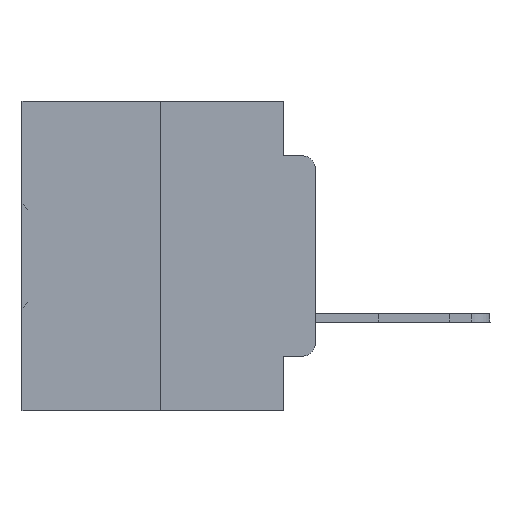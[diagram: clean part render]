
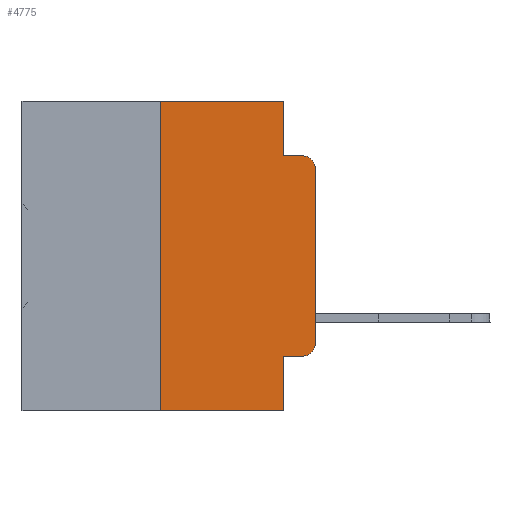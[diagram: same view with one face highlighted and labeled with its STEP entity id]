
A CAD part, left-side view. The second image highlights one B-rep face of the part: STEP entity #4775.
In plain terms, the highlighted planar face has unit normal (-1, 0, 0).
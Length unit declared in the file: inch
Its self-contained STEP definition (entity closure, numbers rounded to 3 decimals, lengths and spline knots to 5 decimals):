
#44 = CARTESIAN_POINT ( 'NONE',  ( 0., 0.25, 0. ) ) ;
#73 = EDGE_CURVE ( 'NONE', #25052, #33834, #27180, .T. ) ;
#574 = VECTOR ( 'NONE', #32646, 39.37008 ) ;
#826 = DIRECTION ( 'NONE',  ( 0., 0., -1. ) ) ;
#978 = ORIENTED_EDGE ( 'NONE', *, *, #10420, .T. ) ;
#1211 = ORIENTED_EDGE ( 'NONE', *, *, #73, .F. ) ;
#1350 = VECTOR ( 'NONE', #23883, 39.37008 ) ;
#1943 = CARTESIAN_POINT ( 'NONE',  ( 0., 0.02, -0.0885 ) ) ;
#2237 = VECTOR ( 'NONE', #25882, 39.37008 ) ;
#2871 = CIRCLE ( 'NONE', #24149, 0.02 ) ;
#3865 = EDGE_CURVE ( 'NONE', #33834, #7707, #8281, .T. ) ;
#3898 = DIRECTION ( 'NONE',  ( 0., 0., -1. ) ) ;
#4092 = PLANE ( 'NONE',  #24202 ) ;
#4153 = CARTESIAN_POINT ( 'NONE',  ( 0., 0.051, 0. ) ) ;
#4378 = VECTOR ( 'NONE', #26690, 39.37008 ) ;
#4775 = ADVANCED_FACE ( 'NONE', ( #29833 ), #4092, .F. ) ;
#5383 = ORIENTED_EDGE ( 'NONE', *, *, #3865, .F. ) ;
#5728 = EDGE_CURVE ( 'NONE', #25775, #24258, #17668, .T. ) ;
#5816 = CARTESIAN_POINT ( 'NONE',  ( 0., 0., -0.1085 ) ) ;
#6337 = CARTESIAN_POINT ( 'NONE',  ( 0., 0.473, 0. ) ) ;
#6495 = ORIENTED_EDGE ( 'NONE', *, *, #21046, .T. ) ;
#6619 = CARTESIAN_POINT ( 'NONE',  ( 0., 0.02, -0.1085 ) ) ;
#7337 = ORIENTED_EDGE ( 'NONE', *, *, #22895, .T. ) ;
#7707 = VERTEX_POINT ( 'NONE', #32157 ) ;
#7719 = VERTEX_POINT ( 'NONE', #21350 ) ;
#7799 = CARTESIAN_POINT ( 'NONE',  ( 0., 0.473, 0. ) ) ;
#8281 = LINE ( 'NONE', #7799, #574 ) ;
#9077 = VERTEX_POINT ( 'NONE', #23490 ) ;
#9442 = VECTOR ( 'NONE', #17511, 39.37008 ) ;
#9446 = LINE ( 'NONE', #31893, #1350 ) ;
#9457 = EDGE_LOOP ( 'NONE', ( #13786, #6495, #19389, #30653, #5383, #1211, #7337, #30926, #978, #21775 ) ) ;
#10019 = CIRCLE ( 'NONE', #19661, 0.02 ) ;
#10065 = VECTOR ( 'NONE', #32995, 39.37008 ) ;
#10070 = CARTESIAN_POINT ( 'NONE',  ( 0., 0., -0.3915 ) ) ;
#10420 = EDGE_CURVE ( 'NONE', #19494, #7719, #27631, .T. ) ;
#12389 = EDGE_CURVE ( 'NONE', #7707, #32078, #19233, .T. ) ;
#12798 = VECTOR ( 'NONE', #826, 39.37008 ) ;
#12874 = EDGE_CURVE ( 'NONE', #7719, #25775, #2871, .T. ) ;
#13786 = ORIENTED_EDGE ( 'NONE', *, *, #5728, .T. ) ;
#14828 = CARTESIAN_POINT ( 'NONE',  ( 0., 0.02, -0.3915 ) ) ;
#15148 = CARTESIAN_POINT ( 'NONE',  ( 0., 0., 0. ) ) ;
#15298 = DIRECTION ( 'NONE',  ( 0., 0., -1. ) ) ;
#16244 = CARTESIAN_POINT ( 'NONE',  ( 0., 0.051, -0.0885 ) ) ;
#17511 = DIRECTION ( 'NONE',  ( 0., 0., 1. ) ) ;
#17525 = DIRECTION ( 'NONE',  ( 0., 0., -1. ) ) ;
#17668 = LINE ( 'NONE', #15148, #2237 ) ;
#18247 = CARTESIAN_POINT ( 'NONE',  ( 0., 0.051, -0.4115 ) ) ;
#18485 = DIRECTION ( 'NONE',  ( 0., -1., 0. ) ) ;
#19233 = LINE ( 'NONE', #4153, #12798 ) ;
#19389 = ORIENTED_EDGE ( 'NONE', *, *, #33827, .F. ) ;
#19494 = VERTEX_POINT ( 'NONE', #27108 ) ;
#19661 = AXIS2_PLACEMENT_3D ( 'NONE', #6619, #20579, #15298 ) ;
#20352 = DIRECTION ( 'NONE',  ( -1., 0., 0. ) ) ;
#20579 = DIRECTION ( 'NONE',  ( -1., 0., 0. ) ) ;
#21046 = EDGE_CURVE ( 'NONE', #24258, #34836, #10019, .T. ) ;
#21350 = CARTESIAN_POINT ( 'NONE',  ( 0., 0.02, -0.4115 ) ) ;
#21775 = ORIENTED_EDGE ( 'NONE', *, *, #12874, .T. ) ;
#22895 = EDGE_CURVE ( 'NONE', #25052, #9077, #9446, .T. ) ;
#23490 = CARTESIAN_POINT ( 'NONE',  ( 0., 0.051, -0.5 ) ) ;
#23883 = DIRECTION ( 'NONE',  ( 0., -1., 0. ) ) ;
#24149 = AXIS2_PLACEMENT_3D ( 'NONE', #14828, #20352, #3898 ) ;
#24202 = AXIS2_PLACEMENT_3D ( 'NONE', #6337, #25616, #17525 ) ;
#24258 = VERTEX_POINT ( 'NONE', #5816 ) ;
#25009 = VECTOR ( 'NONE', #18485, 39.37008 ) ;
#25052 = VERTEX_POINT ( 'NONE', #33846 ) ;
#25616 = DIRECTION ( 'NONE',  ( 1., 0., 0. ) ) ;
#25775 = VERTEX_POINT ( 'NONE', #10070 ) ;
#25882 = DIRECTION ( 'NONE',  ( 0., 0., 1. ) ) ;
#26690 = DIRECTION ( 'NONE',  ( 0., 0., -1. ) ) ;
#27108 = CARTESIAN_POINT ( 'NONE',  ( 0., 0.051, -0.4115 ) ) ;
#27180 = LINE ( 'NONE', #34553, #9442 ) ;
#27232 = CARTESIAN_POINT ( 'NONE',  ( 0., 0.051, -0.0885 ) ) ;
#27631 = LINE ( 'NONE', #18247, #25009 ) ;
#27702 = EDGE_CURVE ( 'NONE', #19494, #9077, #33221, .T. ) ;
#29833 = FACE_OUTER_BOUND ( 'NONE', #9457, .T. ) ;
#30653 = ORIENTED_EDGE ( 'NONE', *, *, #12389, .F. ) ;
#30926 = ORIENTED_EDGE ( 'NONE', *, *, #27702, .F. ) ;
#31893 = CARTESIAN_POINT ( 'NONE',  ( 0., 0.473, -0.5 ) ) ;
#32078 = VERTEX_POINT ( 'NONE', #27232 ) ;
#32157 = CARTESIAN_POINT ( 'NONE',  ( 0., 0.051, 0. ) ) ;
#32646 = DIRECTION ( 'NONE',  ( 0., -1., 0. ) ) ;
#32995 = DIRECTION ( 'NONE',  ( 0., -1., 0. ) ) ;
#33221 = LINE ( 'NONE', #35247, #4378 ) ;
#33827 = EDGE_CURVE ( 'NONE', #32078, #34836, #34210, .T. ) ;
#33834 = VERTEX_POINT ( 'NONE', #44 ) ;
#33846 = CARTESIAN_POINT ( 'NONE',  ( 0., 0.25, -0.5 ) ) ;
#34210 = LINE ( 'NONE', #16244, #10065 ) ;
#34553 = CARTESIAN_POINT ( 'NONE',  ( 0., 0.25, 0. ) ) ;
#34836 = VERTEX_POINT ( 'NONE', #1943 ) ;
#35247 = CARTESIAN_POINT ( 'NONE',  ( 0., 0.051, 0. ) ) ;
